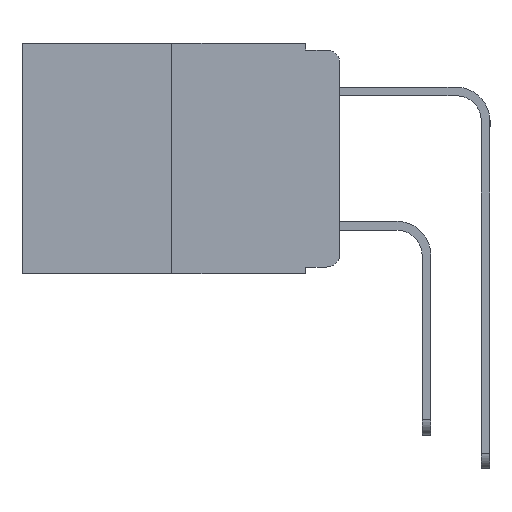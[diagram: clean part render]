
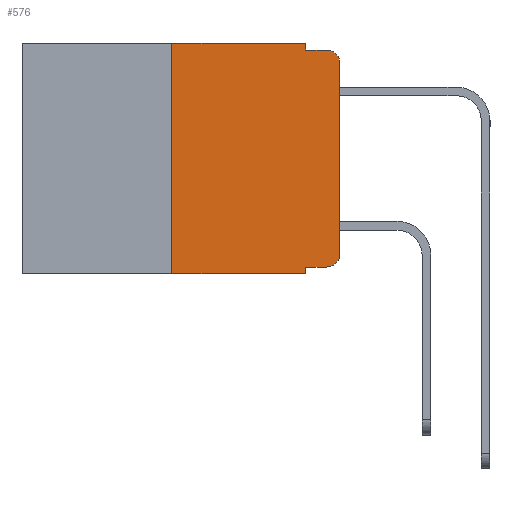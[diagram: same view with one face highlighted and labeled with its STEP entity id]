
A CAD part, left-side view. The second image highlights one B-rep face of the part: STEP entity #576.
In plain terms, the highlighted planar face has unit normal (-1, 0, 0).
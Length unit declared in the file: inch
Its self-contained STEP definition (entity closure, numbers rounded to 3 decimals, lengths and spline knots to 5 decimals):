
#363 = EDGE_LOOP ( 'NONE', ( #11338, #3419, #21059, #9836, #2365, #17295, #4549, #2098, #15494, #17584 ) ) ;
#488 = EDGE_CURVE ( 'NONE', #7080, #782, #9584, .T. ) ;
#576 = ADVANCED_FACE ( 'NONE', ( #21061 ), #1482, .F. ) ;
#596 = CARTESIAN_POINT ( 'NONE',  ( 0., 0.473, -0.343 ) ) ;
#782 = VERTEX_POINT ( 'NONE', #7132 ) ;
#1038 = DIRECTION ( 'NONE',  ( -1., 0., 0. ) ) ;
#1482 = PLANE ( 'NONE',  #13575 ) ;
#1656 = EDGE_CURVE ( 'NONE', #19195, #7080, #13944, .T. ) ;
#2003 = CARTESIAN_POINT ( 'NONE',  ( 0., 0.051, -0.01 ) ) ;
#2042 = VERTEX_POINT ( 'NONE', #11862 ) ;
#2098 = ORIENTED_EDGE ( 'NONE', *, *, #2845, .F. ) ;
#2365 = ORIENTED_EDGE ( 'NONE', *, *, #12882, .F. ) ;
#2845 = EDGE_CURVE ( 'NONE', #19195, #16754, #6623, .T. ) ;
#3026 = CARTESIAN_POINT ( 'NONE',  ( 0., 0.02, -0.01 ) ) ;
#3405 = CARTESIAN_POINT ( 'NONE',  ( 0., 0.051, 0. ) ) ;
#3419 = ORIENTED_EDGE ( 'NONE', *, *, #7491, .T. ) ;
#4010 = EDGE_CURVE ( 'NONE', #11253, #11395, #13818, .T. ) ;
#4528 = VECTOR ( 'NONE', #12451, 39.37008 ) ;
#4549 = ORIENTED_EDGE ( 'NONE', *, *, #15905, .T. ) ;
#4637 = CARTESIAN_POINT ( 'NONE',  ( 0., 0.473, 0. ) ) ;
#4914 = VECTOR ( 'NONE', #14596, 39.37008 ) ;
#5138 = EDGE_CURVE ( 'NONE', #13094, #21508, #6807, .T. ) ;
#5778 = AXIS2_PLACEMENT_3D ( 'NONE', #14522, #8428, #11933 ) ;
#6321 = EDGE_CURVE ( 'NONE', #21508, #13794, #10118, .T. ) ;
#6623 = LINE ( 'NONE', #18990, #19253 ) ;
#6805 = DIRECTION ( 'NONE',  ( 0., 0., -1. ) ) ;
#6807 = LINE ( 'NONE', #18801, #18903 ) ;
#7080 = VERTEX_POINT ( 'NONE', #8550 ) ;
#7132 = CARTESIAN_POINT ( 'NONE',  ( 0., 0., -0.313 ) ) ;
#7491 = EDGE_CURVE ( 'NONE', #2042, #13794, #17116, .T. ) ;
#8031 = LINE ( 'NONE', #19957, #20068 ) ;
#8428 = DIRECTION ( 'NONE',  ( -1., 0., 0. ) ) ;
#8550 = CARTESIAN_POINT ( 'NONE',  ( 0., 0.02, -0.333 ) ) ;
#9202 = CARTESIAN_POINT ( 'NONE',  ( 0., 0.473, 0. ) ) ;
#9537 = CARTESIAN_POINT ( 'NONE',  ( 0., 0.051, -0.01 ) ) ;
#9584 = CIRCLE ( 'NONE', #5778, 0.02 ) ;
#9702 = EDGE_CURVE ( 'NONE', #782, #2042, #8031, .T. ) ;
#9836 = ORIENTED_EDGE ( 'NONE', *, *, #5138, .F. ) ;
#10087 = VECTOR ( 'NONE', #19205, 39.37008 ) ;
#10118 = LINE ( 'NONE', #9537, #14983 ) ;
#11094 = AXIS2_PLACEMENT_3D ( 'NONE', #11225, #1038, #12901 ) ;
#11225 = CARTESIAN_POINT ( 'NONE',  ( 0., 0.02, -0.03 ) ) ;
#11253 = VERTEX_POINT ( 'NONE', #15853 ) ;
#11338 = ORIENTED_EDGE ( 'NONE', *, *, #9702, .T. ) ;
#11395 = VERTEX_POINT ( 'NONE', #19461 ) ;
#11821 = DIRECTION ( 'NONE',  ( 0., 0., -1. ) ) ;
#11862 = CARTESIAN_POINT ( 'NONE',  ( 0., 0., -0.03 ) ) ;
#11933 = DIRECTION ( 'NONE',  ( 0., 0., -1. ) ) ;
#12451 = DIRECTION ( 'NONE',  ( 0., -1., 0. ) ) ;
#12580 = CARTESIAN_POINT ( 'NONE',  ( 0., 0.051, -0.343 ) ) ;
#12882 = EDGE_CURVE ( 'NONE', #11395, #13094, #18966, .T. ) ;
#12901 = DIRECTION ( 'NONE',  ( 0., 0., -1. ) ) ;
#13094 = VERTEX_POINT ( 'NONE', #3405 ) ;
#13575 = AXIS2_PLACEMENT_3D ( 'NONE', #9202, #18266, #6805 ) ;
#13794 = VERTEX_POINT ( 'NONE', #3026 ) ;
#13818 = LINE ( 'NONE', #15032, #4914 ) ;
#13876 = DIRECTION ( 'NONE',  ( 0., 0., -1. ) ) ;
#13944 = LINE ( 'NONE', #16165, #4528 ) ;
#14455 = LINE ( 'NONE', #596, #10087 ) ;
#14522 = CARTESIAN_POINT ( 'NONE',  ( 0., 0.02, -0.313 ) ) ;
#14596 = DIRECTION ( 'NONE',  ( 0., 0., 1. ) ) ;
#14597 = VECTOR ( 'NONE', #14622, 39.37008 ) ;
#14622 = DIRECTION ( 'NONE',  ( 0., -1., 0. ) ) ;
#14983 = VECTOR ( 'NONE', #20937, 39.37008 ) ;
#15032 = CARTESIAN_POINT ( 'NONE',  ( 0., 0.25, 0. ) ) ;
#15494 = ORIENTED_EDGE ( 'NONE', *, *, #1656, .T. ) ;
#15853 = CARTESIAN_POINT ( 'NONE',  ( 0., 0.25, -0.343 ) ) ;
#15905 = EDGE_CURVE ( 'NONE', #11253, #16754, #14455, .T. ) ;
#16165 = CARTESIAN_POINT ( 'NONE',  ( 0., 0.051, -0.333 ) ) ;
#16372 = CARTESIAN_POINT ( 'NONE',  ( 0., 0.051, -0.333 ) ) ;
#16754 = VERTEX_POINT ( 'NONE', #12580 ) ;
#17116 = CIRCLE ( 'NONE', #11094, 0.02 ) ;
#17295 = ORIENTED_EDGE ( 'NONE', *, *, #4010, .F. ) ;
#17584 = ORIENTED_EDGE ( 'NONE', *, *, #488, .T. ) ;
#18266 = DIRECTION ( 'NONE',  ( 1., 0., 0. ) ) ;
#18801 = CARTESIAN_POINT ( 'NONE',  ( 0., 0.051, 0. ) ) ;
#18903 = VECTOR ( 'NONE', #13876, 39.37008 ) ;
#18966 = LINE ( 'NONE', #4637, #14597 ) ;
#18990 = CARTESIAN_POINT ( 'NONE',  ( 0., 0.051, 0. ) ) ;
#19195 = VERTEX_POINT ( 'NONE', #16372 ) ;
#19205 = DIRECTION ( 'NONE',  ( 0., -1., 0. ) ) ;
#19253 = VECTOR ( 'NONE', #11821, 39.37008 ) ;
#19461 = CARTESIAN_POINT ( 'NONE',  ( 0., 0.25, 0. ) ) ;
#19957 = CARTESIAN_POINT ( 'NONE',  ( 0., 0., 0. ) ) ;
#20068 = VECTOR ( 'NONE', #21562, 39.37008 ) ;
#20937 = DIRECTION ( 'NONE',  ( 0., -1., 0. ) ) ;
#21059 = ORIENTED_EDGE ( 'NONE', *, *, #6321, .F. ) ;
#21061 = FACE_OUTER_BOUND ( 'NONE', #363, .T. ) ;
#21508 = VERTEX_POINT ( 'NONE', #2003 ) ;
#21562 = DIRECTION ( 'NONE',  ( 0., 0., 1. ) ) ;
